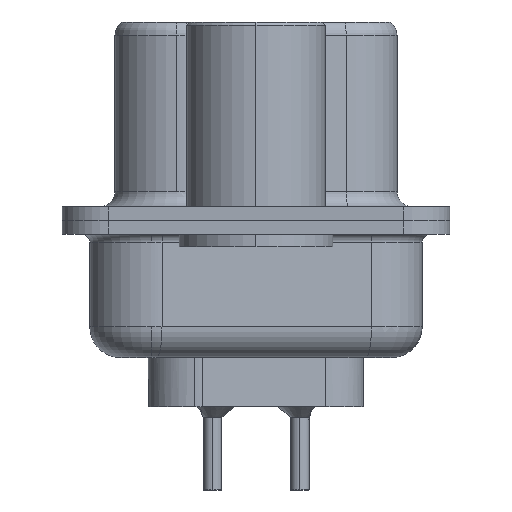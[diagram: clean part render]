
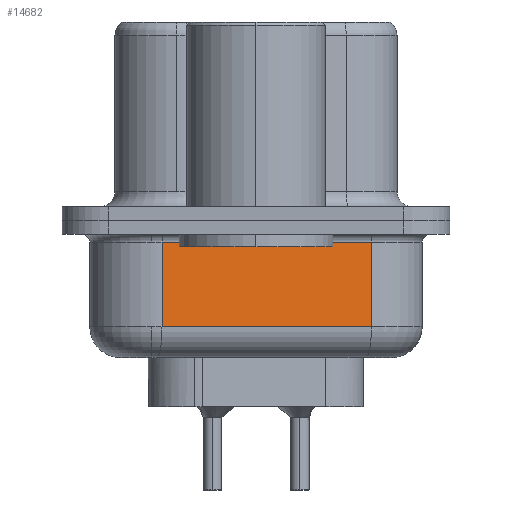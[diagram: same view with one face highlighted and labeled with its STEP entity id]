
A CAD part, left-side view. The second image highlights one B-rep face of the part: STEP entity #14682.
In plain terms, the highlighted planar face has unit normal (-0.985, -0.174, 0).
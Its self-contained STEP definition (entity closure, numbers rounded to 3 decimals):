
#828 = DIRECTION ( 'NONE',  ( 0., 0., 1. ) ) ;
#1009 = CARTESIAN_POINT ( 'NONE',  ( 2.875, 3.053, -4.45 ) ) ;
#1010 = CARTESIAN_POINT ( 'NONE',  ( 4.074, -3.747, -0.7 ) ) ;
#1314 = ORIENTED_EDGE ( 'NONE', *, *, #4705, .F. ) ;
#1648 = AXIS2_PLACEMENT_3D ( 'NONE', #1009, #11502, #2511 ) ;
#2068 = EDGE_CURVE ( 'NONE', #9972, #6615, #18943, .T. ) ;
#2158 = DIRECTION ( 'NONE',  ( -0.174, 0.985, 0. ) ) ;
#2511 = DIRECTION ( 'NONE',  ( -0.174, 0.985, 0. ) ) ;
#2604 = ORIENTED_EDGE ( 'NONE', *, *, #4086, .T. ) ;
#3198 = EDGE_CURVE ( 'NONE', #15739, #9972, #7978, .T. ) ;
#4086 = EDGE_CURVE ( 'NONE', #6615, #14743, #10506, .T. ) ;
#4705 = EDGE_CURVE ( 'NONE', #15739, #14743, #6566, .T. ) ;
#5913 = DIRECTION ( 'NONE',  ( 0.174, -0.985, 0. ) ) ;
#6124 = VECTOR ( 'NONE', #8253, 1000. ) ;
#6566 = LINE ( 'NONE', #18772, #17954 ) ;
#6615 = VERTEX_POINT ( 'NONE', #1010 ) ;
#6694 = CARTESIAN_POINT ( 'NONE',  ( 2.875, 3.053, -0.7 ) ) ;
#7497 = VECTOR ( 'NONE', #5913, 1000. ) ;
#7978 = LINE ( 'NONE', #8907, #7497 ) ;
#8253 = DIRECTION ( 'NONE',  ( 0., 0., 1. ) ) ;
#8397 = FACE_OUTER_BOUND ( 'NONE', #12084, .T. ) ;
#8907 = CARTESIAN_POINT ( 'NONE',  ( 2.875, 3.053, -3.45 ) ) ;
#9972 = VERTEX_POINT ( 'NONE', #13738 ) ;
#10012 = PLANE ( 'NONE',  #1648 ) ;
#10506 = LINE ( 'NONE', #6694, #18912 ) ;
#11280 = CARTESIAN_POINT ( 'NONE',  ( 4.074, -3.747, -4.45 ) ) ;
#11502 = DIRECTION ( 'NONE',  ( 0.985, 0.174, 0. ) ) ;
#12084 = EDGE_LOOP ( 'NONE', ( #1314, #16885, #12202, #2604 ) ) ;
#12202 = ORIENTED_EDGE ( 'NONE', *, *, #2068, .T. ) ;
#13738 = CARTESIAN_POINT ( 'NONE',  ( 4.074, -3.747, -3.45 ) ) ;
#14031 = CARTESIAN_POINT ( 'NONE',  ( 2.875, 3.053, -3.45 ) ) ;
#14682 = ADVANCED_FACE ( 'NONE', ( #8397 ), #10012, .F. ) ;
#14743 = VERTEX_POINT ( 'NONE', #16067 ) ;
#15739 = VERTEX_POINT ( 'NONE', #14031 ) ;
#16067 = CARTESIAN_POINT ( 'NONE',  ( 2.875, 3.053, -0.7 ) ) ;
#16885 = ORIENTED_EDGE ( 'NONE', *, *, #3198, .T. ) ;
#17954 = VECTOR ( 'NONE', #828, 1000. ) ;
#18772 = CARTESIAN_POINT ( 'NONE',  ( 2.875, 3.053, -4.45 ) ) ;
#18912 = VECTOR ( 'NONE', #2158, 1000. ) ;
#18943 = LINE ( 'NONE', #11280, #6124 ) ;
